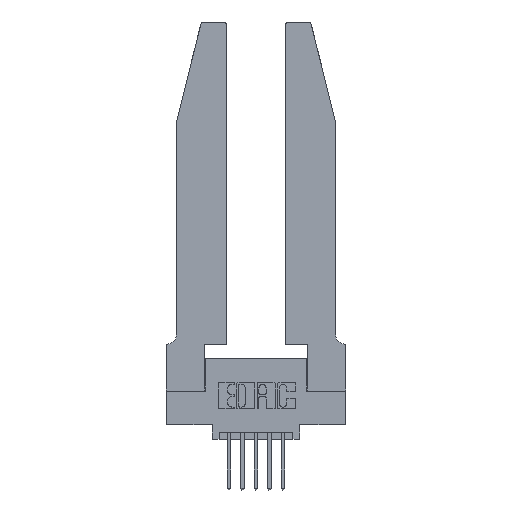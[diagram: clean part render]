
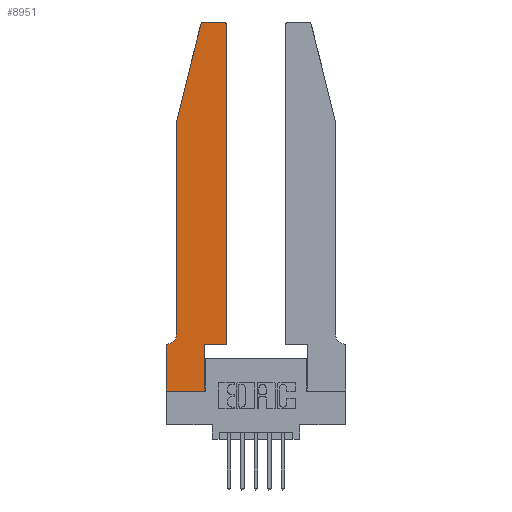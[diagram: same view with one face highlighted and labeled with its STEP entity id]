
A CAD part, top view. The second image highlights one B-rep face of the part: STEP entity #8951.
In plain terms, the highlighted planar face has unit normal (0, 0, 1).
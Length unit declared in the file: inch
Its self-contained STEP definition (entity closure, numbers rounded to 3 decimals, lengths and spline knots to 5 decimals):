
#88 = CARTESIAN_POINT ( 'NONE',  ( 0.2865, 0., 0.37 ) ) ;
#181 = VERTEX_POINT ( 'NONE', #353 ) ;
#240 = ORIENTED_EDGE ( 'NONE', *, *, #7680, .T. ) ;
#353 = CARTESIAN_POINT ( 'NONE',  ( 0., 0., 0.37 ) ) ;
#463 = ORIENTED_EDGE ( 'NONE', *, *, #3138, .T. ) ;
#650 = ORIENTED_EDGE ( 'NONE', *, *, #12836, .T. ) ;
#726 = ORIENTED_EDGE ( 'NONE', *, *, #5555, .T. ) ;
#899 = EDGE_CURVE ( 'NONE', #5319, #910, #1169, .T. ) ;
#910 = VERTEX_POINT ( 'NONE', #5121 ) ;
#973 = CARTESIAN_POINT ( 'NONE',  ( 0.4505, 0.35, 0.37 ) ) ;
#1092 = CIRCLE ( 'NONE', #3133, 0.03 ) ;
#1133 = VERTEX_POINT ( 'NONE', #6483 ) ;
#1169 = LINE ( 'NONE', #6236, #12523 ) ;
#1210 = CARTESIAN_POINT ( 'NONE',  ( 0.2605, 2.75, 0.37 ) ) ;
#1449 = CARTESIAN_POINT ( 'NONE',  ( 0.284, 2.72, 0.37 ) ) ;
#1660 = ORIENTED_EDGE ( 'NONE', *, *, #3460, .T. ) ;
#1815 = ORIENTED_EDGE ( 'NONE', *, *, #899, .T. ) ;
#1890 = EDGE_CURVE ( 'NONE', #9176, #2384, #4734, .T. ) ;
#1993 = LINE ( 'NONE', #6034, #10173 ) ;
#2048 = DIRECTION ( 'NONE',  ( 0., 0., 1. ) ) ;
#2062 = DIRECTION ( 'NONE',  ( 1., 0., 0. ) ) ;
#2124 = DIRECTION ( 'NONE',  ( 0., 1., 0. ) ) ;
#2200 = EDGE_CURVE ( 'NONE', #8587, #8455, #6709, .T. ) ;
#2211 = VERTEX_POINT ( 'NONE', #12541 ) ;
#2360 = DIRECTION ( 'NONE',  ( -1., 0., 0. ) ) ;
#2384 = VERTEX_POINT ( 'NONE', #9468 ) ;
#2483 = CARTESIAN_POINT ( 'NONE',  ( 0.4205, 2.72, 0.37 ) ) ;
#2592 = DIRECTION ( 'NONE',  ( 1., 0., 0. ) ) ;
#3133 = AXIS2_PLACEMENT_3D ( 'NONE', #1449, #8930, #2592 ) ;
#3138 = EDGE_CURVE ( 'NONE', #13574, #12752, #10199, .T. ) ;
#3173 = ORIENTED_EDGE ( 'NONE', *, *, #6379, .T. ) ;
#3256 = ORIENTED_EDGE ( 'NONE', *, *, #6802, .T. ) ;
#3460 = EDGE_CURVE ( 'NONE', #8455, #5319, #9349, .T. ) ;
#3730 = LINE ( 'NONE', #973, #9000 ) ;
#3735 = DIRECTION ( 'NONE',  ( -1., 0., 0. ) ) ;
#3753 = DIRECTION ( 'NONE',  ( 0., 0., -1. ) ) ;
#3796 = CARTESIAN_POINT ( 'NONE',  ( 0.0055, 0.42, 0.37 ) ) ;
#3840 = CARTESIAN_POINT ( 'NONE',  ( 0., 0., 0.37 ) ) ;
#3869 = VERTEX_POINT ( 'NONE', #88 ) ;
#3912 = CARTESIAN_POINT ( 'NONE',  ( 0.2865, 0.35, 0.37 ) ) ;
#4398 = CARTESIAN_POINT ( 'NONE',  ( 0.2865, 0.35, 0.37 ) ) ;
#4495 = EDGE_CURVE ( 'NONE', #910, #181, #8167, .T. ) ;
#4671 = LINE ( 'NONE', #4398, #7476 ) ;
#4734 = CIRCLE ( 'NONE', #10751, 0.03 ) ;
#4936 = CARTESIAN_POINT ( 'NONE',  ( 0., 0.35, 0.37 ) ) ;
#5121 = CARTESIAN_POINT ( 'NONE',  ( 0., 0.35, 0.37 ) ) ;
#5219 = CARTESIAN_POINT ( 'NONE',  ( 0.0055, 0.35, 0.37 ) ) ;
#5319 = VERTEX_POINT ( 'NONE', #5219 ) ;
#5463 = ORIENTED_EDGE ( 'NONE', *, *, #6548, .T. ) ;
#5555 = EDGE_CURVE ( 'NONE', #2384, #1133, #13385, .T. ) ;
#5647 = DIRECTION ( 'NONE',  ( -1., 0., 0. ) ) ;
#5776 = FACE_OUTER_BOUND ( 'NONE', #12470, .T. ) ;
#5950 = DIRECTION ( 'NONE',  ( 1., 0., 0. ) ) ;
#5985 = LINE ( 'NONE', #3840, #8452 ) ;
#6016 = DIRECTION ( 'NONE',  ( 1., 0., 0. ) ) ;
#6034 = CARTESIAN_POINT ( 'NONE',  ( 0.0755, 2., 0.37 ) ) ;
#6176 = AXIS2_PLACEMENT_3D ( 'NONE', #4936, #12330, #6016 ) ;
#6236 = CARTESIAN_POINT ( 'NONE',  ( 0.0755, 0.35, 0.37 ) ) ;
#6291 = CARTESIAN_POINT ( 'NONE',  ( 0.4505, 0.35, 0.37 ) ) ;
#6379 = EDGE_CURVE ( 'NONE', #1133, #2211, #1092, .T. ) ;
#6483 = CARTESIAN_POINT ( 'NONE',  ( 0.284, 2.75, 0.37 ) ) ;
#6548 = EDGE_CURVE ( 'NONE', #2211, #8587, #1993, .T. ) ;
#6709 = LINE ( 'NONE', #12676, #9547 ) ;
#6744 = ORIENTED_EDGE ( 'NONE', *, *, #1890, .T. ) ;
#6802 = EDGE_CURVE ( 'NONE', #3869, #13574, #4671, .T. ) ;
#7131 = VECTOR ( 'NONE', #2360, 39.37008 ) ;
#7476 = VECTOR ( 'NONE', #11799, 39.37008 ) ;
#7680 = EDGE_CURVE ( 'NONE', #181, #3869, #5985, .T. ) ;
#8167 = LINE ( 'NONE', #10829, #13414 ) ;
#8279 = CARTESIAN_POINT ( 'NONE',  ( 0.0755, 0.42, 0.37 ) ) ;
#8418 = DIRECTION ( 'NONE',  ( 1., 0., 0. ) ) ;
#8452 = VECTOR ( 'NONE', #5950, 39.37008 ) ;
#8455 = VERTEX_POINT ( 'NONE', #8279 ) ;
#8587 = VERTEX_POINT ( 'NONE', #9588 ) ;
#8659 = AXIS2_PLACEMENT_3D ( 'NONE', #3796, #3753, #3735 ) ;
#8803 = ORIENTED_EDGE ( 'NONE', *, *, #2200, .T. ) ;
#8839 = CARTESIAN_POINT ( 'NONE',  ( 0.4505, 0.35, 0.37 ) ) ;
#8930 = DIRECTION ( 'NONE',  ( 0., 0., 1. ) ) ;
#8951 = ADVANCED_FACE ( 'NONE', ( #5776 ), #11254, .T. ) ;
#9000 = VECTOR ( 'NONE', #2124, 39.37008 ) ;
#9176 = VERTEX_POINT ( 'NONE', #9902 ) ;
#9349 = CIRCLE ( 'NONE', #8659, 0.07 ) ;
#9468 = CARTESIAN_POINT ( 'NONE',  ( 0.4205, 2.75, 0.37 ) ) ;
#9547 = VECTOR ( 'NONE', #13035, 39.37008 ) ;
#9588 = CARTESIAN_POINT ( 'NONE',  ( 0.0755, 2., 0.37 ) ) ;
#9861 = ORIENTED_EDGE ( 'NONE', *, *, #4495, .T. ) ;
#9902 = CARTESIAN_POINT ( 'NONE',  ( 0.4505, 2.72, 0.37 ) ) ;
#10173 = VECTOR ( 'NONE', #10260, 39.37008 ) ;
#10199 = LINE ( 'NONE', #8839, #12310 ) ;
#10260 = DIRECTION ( 'NONE',  ( -0.239, -0.971, 0. ) ) ;
#10751 = AXIS2_PLACEMENT_3D ( 'NONE', #2483, #2048, #2062 ) ;
#10829 = CARTESIAN_POINT ( 'NONE',  ( 0., 0., 0.37 ) ) ;
#11254 = PLANE ( 'NONE',  #6176 ) ;
#11799 = DIRECTION ( 'NONE',  ( 0., 1., 0. ) ) ;
#12310 = VECTOR ( 'NONE', #8418, 39.37008 ) ;
#12330 = DIRECTION ( 'NONE',  ( 0., 0., 1. ) ) ;
#12470 = EDGE_LOOP ( 'NONE', ( #726, #3173, #5463, #8803, #1660, #1815, #9861, #240, #3256, #463, #650, #6744 ) ) ;
#12523 = VECTOR ( 'NONE', #5647, 39.37008 ) ;
#12541 = CARTESIAN_POINT ( 'NONE',  ( 0.25487, 2.72718, 0.37 ) ) ;
#12676 = CARTESIAN_POINT ( 'NONE',  ( 0.0755, 2., 0.37 ) ) ;
#12752 = VERTEX_POINT ( 'NONE', #6291 ) ;
#12836 = EDGE_CURVE ( 'NONE', #12752, #9176, #3730, .T. ) ;
#12881 = DIRECTION ( 'NONE',  ( 0., -1., 0. ) ) ;
#13035 = DIRECTION ( 'NONE',  ( 0., -1., 0. ) ) ;
#13385 = LINE ( 'NONE', #1210, #7131 ) ;
#13414 = VECTOR ( 'NONE', #12881, 39.37008 ) ;
#13574 = VERTEX_POINT ( 'NONE', #3912 ) ;
